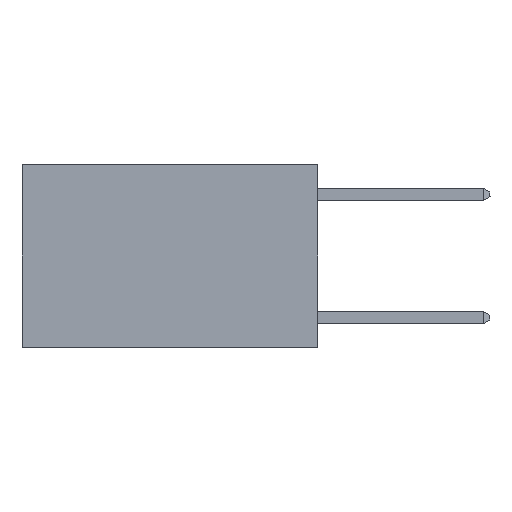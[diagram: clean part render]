
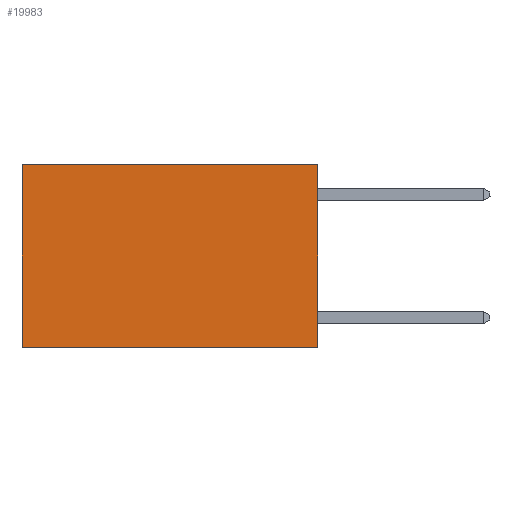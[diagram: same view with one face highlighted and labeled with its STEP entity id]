
A CAD part, left-side view. The second image highlights one B-rep face of the part: STEP entity #19983.
In plain terms, the highlighted planar face has unit normal (-1, 0, 0).
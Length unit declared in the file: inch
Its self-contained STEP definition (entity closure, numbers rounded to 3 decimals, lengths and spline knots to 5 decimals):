
#935 = CARTESIAN_POINT ( 'NONE',  ( 0.2625, 0., -0.37 ) ) ;
#2153 = DIRECTION ( 'NONE',  ( 0., 0., -1. ) ) ;
#3056 = CARTESIAN_POINT ( 'NONE',  ( 0.2625, 0.6, -0.37 ) ) ;
#4107 = CARTESIAN_POINT ( 'NONE',  ( 0.2625, 0., 0. ) ) ;
#5318 = LINE ( 'NONE', #12121, #15571 ) ;
#5861 = LINE ( 'NONE', #935, #17242 ) ;
#6098 = EDGE_CURVE ( 'NONE', #18538, #21754, #13108, .T. ) ;
#6189 = EDGE_LOOP ( 'NONE', ( #13325, #11649, #10860, #11592 ) ) ;
#6448 = DIRECTION ( 'NONE',  ( 0., 0., -1. ) ) ;
#6602 = EDGE_CURVE ( 'NONE', #21754, #13175, #5861, .T. ) ;
#7006 = CARTESIAN_POINT ( 'NONE',  ( 0.2625, 0.6, 0. ) ) ;
#8099 = CARTESIAN_POINT ( 'NONE',  ( 0.2625, 0., 0. ) ) ;
#8756 = VECTOR ( 'NONE', #10895, 39.37008 ) ;
#10516 = PLANE ( 'NONE',  #21552 ) ;
#10860 = ORIENTED_EDGE ( 'NONE', *, *, #6098, .F. ) ;
#10895 = DIRECTION ( 'NONE',  ( 0., 1., 0. ) ) ;
#11422 = DIRECTION ( 'NONE',  ( 0., 1., 0. ) ) ;
#11592 = ORIENTED_EDGE ( 'NONE', *, *, #17983, .T. ) ;
#11649 = ORIENTED_EDGE ( 'NONE', *, *, #6602, .F. ) ;
#11723 = CARTESIAN_POINT ( 'NONE',  ( 0.2625, 0., 0. ) ) ;
#12121 = CARTESIAN_POINT ( 'NONE',  ( 0.2625, 0.6, 0. ) ) ;
#13108 = LINE ( 'NONE', #8099, #14561 ) ;
#13175 = VERTEX_POINT ( 'NONE', #3056 ) ;
#13325 = ORIENTED_EDGE ( 'NONE', *, *, #14230, .T. ) ;
#14230 = EDGE_CURVE ( 'NONE', #19194, #13175, #5318, .T. ) ;
#14288 = CARTESIAN_POINT ( 'NONE',  ( 0.2625, 0., -0.37 ) ) ;
#14561 = VECTOR ( 'NONE', #6448, 39.37008 ) ;
#15571 = VECTOR ( 'NONE', #16104, 39.37008 ) ;
#16104 = DIRECTION ( 'NONE',  ( 0., 0., -1. ) ) ;
#17242 = VECTOR ( 'NONE', #11422, 39.37008 ) ;
#17983 = EDGE_CURVE ( 'NONE', #18538, #19194, #19319, .T. ) ;
#18538 = VERTEX_POINT ( 'NONE', #11723 ) ;
#18952 = FACE_OUTER_BOUND ( 'NONE', #6189, .T. ) ;
#19194 = VERTEX_POINT ( 'NONE', #7006 ) ;
#19319 = LINE ( 'NONE', #4107, #8756 ) ;
#19983 = ADVANCED_FACE ( 'NONE', ( #18952 ), #10516, .F. ) ;
#20404 = CARTESIAN_POINT ( 'NONE',  ( 0.2625, 0., 0. ) ) ;
#20852 = DIRECTION ( 'NONE',  ( 1., 0., 0. ) ) ;
#21552 = AXIS2_PLACEMENT_3D ( 'NONE', #20404, #20852, #2153 ) ;
#21754 = VERTEX_POINT ( 'NONE', #14288 ) ;
